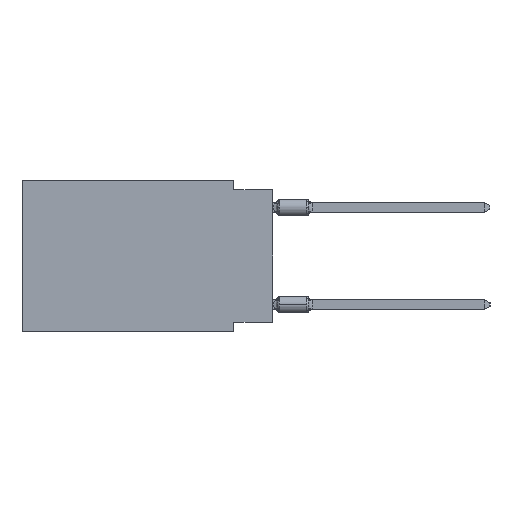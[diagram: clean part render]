
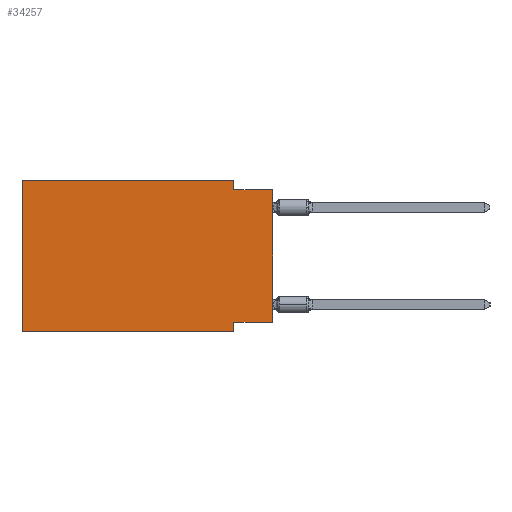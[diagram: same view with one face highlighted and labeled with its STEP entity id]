
A CAD part, left-side view. The second image highlights one B-rep face of the part: STEP entity #34257.
In plain terms, the highlighted planar face has unit normal (-1, 0, 0).
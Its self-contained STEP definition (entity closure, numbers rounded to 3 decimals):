
#329 = EDGE_CURVE ( 'NONE', #6456, #36787, #12374, .T. ) ;
#1759 = CARTESIAN_POINT ( 'NONE',  ( 0., 0., -0.635 ) ) ;
#3213 = VECTOR ( 'NONE', #43371, 1000. ) ;
#3524 = CARTESIAN_POINT ( 'NONE',  ( 0., 16.383, -9.906 ) ) ;
#5166 = VECTOR ( 'NONE', #38258, 1000. ) ;
#5497 = ORIENTED_EDGE ( 'NONE', *, *, #8504, .T. ) ;
#6456 = VERTEX_POINT ( 'NONE', #23115 ) ;
#6703 = CARTESIAN_POINT ( 'NONE',  ( 0., 16.383, 0. ) ) ;
#6792 = CARTESIAN_POINT ( 'NONE',  ( 0., 2.54, -9.271 ) ) ;
#6830 = DIRECTION ( 'NONE',  ( 0., -1., 0. ) ) ;
#7284 = LINE ( 'NONE', #34941, #29300 ) ;
#8504 = EDGE_CURVE ( 'NONE', #31820, #21233, #23644, .T. ) ;
#9417 = ORIENTED_EDGE ( 'NONE', *, *, #28126, .F. ) ;
#9609 = VERTEX_POINT ( 'NONE', #1759 ) ;
#11317 = VERTEX_POINT ( 'NONE', #6792 ) ;
#11925 = AXIS2_PLACEMENT_3D ( 'NONE', #6703, #39936, #43255 ) ;
#12374 = LINE ( 'NONE', #25664, #42529 ) ;
#12755 = DIRECTION ( 'NONE',  ( 0., 1., 0. ) ) ;
#13011 = CARTESIAN_POINT ( 'NONE',  ( 0., 2.54, -0.635 ) ) ;
#13712 = EDGE_CURVE ( 'NONE', #14295, #6456, #34205, .T. ) ;
#14295 = VERTEX_POINT ( 'NONE', #33624 ) ;
#15534 = EDGE_LOOP ( 'NONE', ( #27879, #34358, #30993, #39327, #30819, #5497, #31124, #9417 ) ) ;
#15543 = VERTEX_POINT ( 'NONE', #32356 ) ;
#15969 = CARTESIAN_POINT ( 'NONE',  ( 0., 2.54, -9.906 ) ) ;
#17145 = EDGE_CURVE ( 'NONE', #31820, #14295, #28767, .T. ) ;
#17373 = DIRECTION ( 'NONE',  ( 0., -1., 0. ) ) ;
#19013 = DIRECTION ( 'NONE',  ( 0., 0., -1. ) ) ;
#19458 = DIRECTION ( 'NONE',  ( 0., 0., 1. ) ) ;
#19839 = LINE ( 'NONE', #39795, #39377 ) ;
#20545 = LINE ( 'NONE', #41158, #5166 ) ;
#20773 = DIRECTION ( 'NONE',  ( 0., -1., 0. ) ) ;
#21233 = VERTEX_POINT ( 'NONE', #15969 ) ;
#23115 = CARTESIAN_POINT ( 'NONE',  ( 0., 2.54, 0. ) ) ;
#23644 = LINE ( 'NONE', #37160, #39854 ) ;
#25664 = CARTESIAN_POINT ( 'NONE',  ( 0., 2.54, 0. ) ) ;
#26187 = PLANE ( 'NONE',  #11925 ) ;
#27227 = VECTOR ( 'NONE', #19458, 1000. ) ;
#27879 = ORIENTED_EDGE ( 'NONE', *, *, #33374, .T. ) ;
#28126 = EDGE_CURVE ( 'NONE', #15543, #11317, #19839, .T. ) ;
#28767 = LINE ( 'NONE', #28979, #27227 ) ;
#28979 = CARTESIAN_POINT ( 'NONE',  ( 0., 16.383, 0. ) ) ;
#29216 = EDGE_CURVE ( 'NONE', #11317, #21233, #20545, .T. ) ;
#29300 = VECTOR ( 'NONE', #20773, 1000. ) ;
#30819 = ORIENTED_EDGE ( 'NONE', *, *, #17145, .F. ) ;
#30886 = CARTESIAN_POINT ( 'NONE',  ( 0., 16.383, 0. ) ) ;
#30993 = ORIENTED_EDGE ( 'NONE', *, *, #329, .F. ) ;
#31124 = ORIENTED_EDGE ( 'NONE', *, *, #29216, .F. ) ;
#31820 = VERTEX_POINT ( 'NONE', #3524 ) ;
#31995 = EDGE_CURVE ( 'NONE', #36787, #9609, #7284, .T. ) ;
#32356 = CARTESIAN_POINT ( 'NONE',  ( 0., 0., -9.271 ) ) ;
#33374 = EDGE_CURVE ( 'NONE', #15543, #9609, #33601, .T. ) ;
#33601 = LINE ( 'NONE', #43798, #3213 ) ;
#33624 = CARTESIAN_POINT ( 'NONE',  ( 0., 16.383, 0. ) ) ;
#34205 = LINE ( 'NONE', #30886, #37634 ) ;
#34257 = ADVANCED_FACE ( 'NONE', ( #43039 ), #26187, .F. ) ;
#34358 = ORIENTED_EDGE ( 'NONE', *, *, #31995, .F. ) ;
#34941 = CARTESIAN_POINT ( 'NONE',  ( 0., 0., -0.635 ) ) ;
#36787 = VERTEX_POINT ( 'NONE', #13011 ) ;
#37160 = CARTESIAN_POINT ( 'NONE',  ( 0., 16.383, -9.906 ) ) ;
#37634 = VECTOR ( 'NONE', #17373, 1000. ) ;
#38258 = DIRECTION ( 'NONE',  ( 0., 0., -1. ) ) ;
#39327 = ORIENTED_EDGE ( 'NONE', *, *, #13712, .F. ) ;
#39377 = VECTOR ( 'NONE', #12755, 1000. ) ;
#39795 = CARTESIAN_POINT ( 'NONE',  ( 0., 0., -9.271 ) ) ;
#39854 = VECTOR ( 'NONE', #6830, 1000. ) ;
#39936 = DIRECTION ( 'NONE',  ( 1., 0., 0. ) ) ;
#41158 = CARTESIAN_POINT ( 'NONE',  ( 0., 2.54, -9.906 ) ) ;
#42529 = VECTOR ( 'NONE', #19013, 1000. ) ;
#43039 = FACE_OUTER_BOUND ( 'NONE', #15534, .T. ) ;
#43255 = DIRECTION ( 'NONE',  ( 0., 0., -1. ) ) ;
#43371 = DIRECTION ( 'NONE',  ( 0., 0., 1. ) ) ;
#43798 = CARTESIAN_POINT ( 'NONE',  ( 0., 0., 0. ) ) ;
